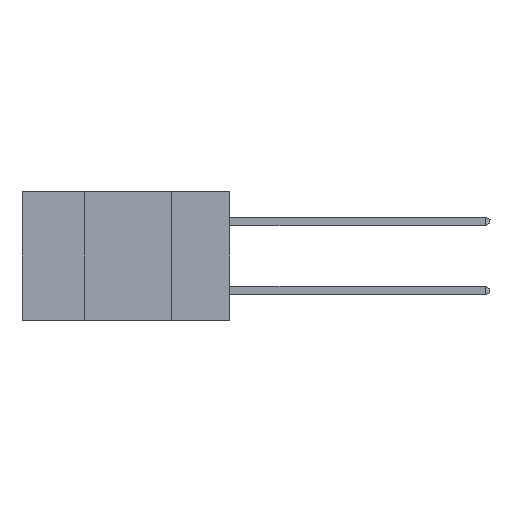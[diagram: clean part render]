
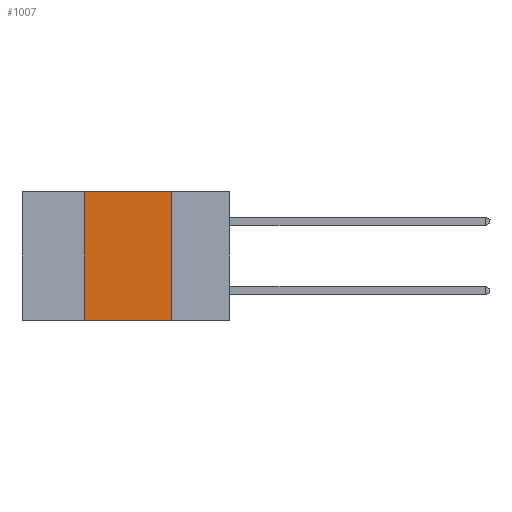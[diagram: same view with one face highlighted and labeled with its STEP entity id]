
A CAD part, left-side view. The second image highlights one B-rep face of the part: STEP entity #1007.
In plain terms, the highlighted planar face has unit normal (-1, 0, 0).
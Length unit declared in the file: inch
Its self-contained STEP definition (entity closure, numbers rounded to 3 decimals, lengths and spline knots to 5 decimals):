
#86 = EDGE_CURVE ( 'NONE', #13922, #121, #5762, .T. ) ;
#121 = VERTEX_POINT ( 'NONE', #8807 ) ;
#214 = VECTOR ( 'NONE', #9945, 39.37008 ) ;
#697 = LINE ( 'NONE', #6011, #3009 ) ;
#772 = EDGE_CURVE ( 'NONE', #13922, #10000, #697, .T. ) ;
#1007 = ADVANCED_FACE ( 'NONE', ( #2676 ), #13411, .F. ) ;
#1465 = DIRECTION ( 'NONE',  ( 1., 0., 0. ) ) ;
#2103 = VECTOR ( 'NONE', #16417, 39.37008 ) ;
#2676 = FACE_OUTER_BOUND ( 'NONE', #8930, .T. ) ;
#2822 = EDGE_CURVE ( 'NONE', #3411, #10000, #10043, .T. ) ;
#2854 = CARTESIAN_POINT ( 'NONE',  ( 0., 0.42, -0.37 ) ) ;
#3009 = VECTOR ( 'NONE', #11324, 39.37008 ) ;
#3321 = CARTESIAN_POINT ( 'NONE',  ( 0., 0.17, -0.37 ) ) ;
#3411 = VERTEX_POINT ( 'NONE', #6328 ) ;
#4047 = ORIENTED_EDGE ( 'NONE', *, *, #772, .T. ) ;
#4760 = ORIENTED_EDGE ( 'NONE', *, *, #2822, .F. ) ;
#5762 = LINE ( 'NONE', #11082, #2103 ) ;
#6011 = CARTESIAN_POINT ( 'NONE',  ( 0., 0.6, -0.37 ) ) ;
#6246 = CARTESIAN_POINT ( 'NONE',  ( 0., 0.6, 0. ) ) ;
#6328 = CARTESIAN_POINT ( 'NONE',  ( 0., 0.17, 0. ) ) ;
#6928 = VECTOR ( 'NONE', #11300, 39.37008 ) ;
#7379 = LINE ( 'NONE', #6246, #6928 ) ;
#8156 = CARTESIAN_POINT ( 'NONE',  ( 0., 0.17, -0.37 ) ) ;
#8807 = CARTESIAN_POINT ( 'NONE',  ( 0., 0.42, 0. ) ) ;
#8930 = EDGE_LOOP ( 'NONE', ( #4760, #15254, #12216, #4047 ) ) ;
#9945 = DIRECTION ( 'NONE',  ( 0., 0., -1. ) ) ;
#10000 = VERTEX_POINT ( 'NONE', #8156 ) ;
#10043 = LINE ( 'NONE', #3321, #214 ) ;
#11082 = CARTESIAN_POINT ( 'NONE',  ( 0., 0.42, -0.37 ) ) ;
#11300 = DIRECTION ( 'NONE',  ( 0., -1., 0. ) ) ;
#11324 = DIRECTION ( 'NONE',  ( 0., -1., 0. ) ) ;
#12216 = ORIENTED_EDGE ( 'NONE', *, *, #86, .F. ) ;
#13411 = PLANE ( 'NONE',  #15184 ) ;
#13577 = CARTESIAN_POINT ( 'NONE',  ( 0., 0.6, 0. ) ) ;
#13922 = VERTEX_POINT ( 'NONE', #2854 ) ;
#14119 = EDGE_CURVE ( 'NONE', #121, #3411, #7379, .T. ) ;
#14810 = DIRECTION ( 'NONE',  ( 0., 0., -1. ) ) ;
#15184 = AXIS2_PLACEMENT_3D ( 'NONE', #13577, #1465, #14810 ) ;
#15254 = ORIENTED_EDGE ( 'NONE', *, *, #14119, .F. ) ;
#16417 = DIRECTION ( 'NONE',  ( 0., 0., 1. ) ) ;
